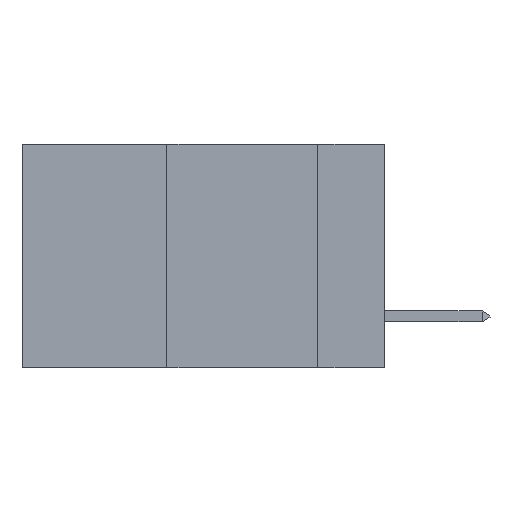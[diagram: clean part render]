
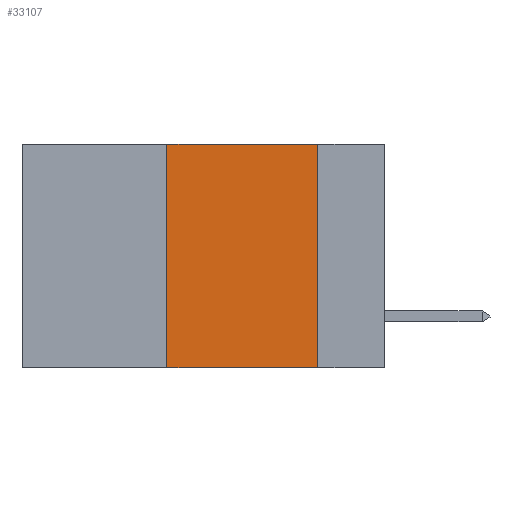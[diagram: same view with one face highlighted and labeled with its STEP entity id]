
A CAD part, left-side view. The second image highlights one B-rep face of the part: STEP entity #33107.
In plain terms, the highlighted planar face has unit normal (-1, 0, 0).
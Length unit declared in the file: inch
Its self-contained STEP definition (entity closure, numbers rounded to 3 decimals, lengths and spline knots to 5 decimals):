
#845 = CARTESIAN_POINT ( 'NONE',  ( 0., 0.6, -0.37 ) ) ;
#1303 = DIRECTION ( 'NONE',  ( 1., 0., 0. ) ) ;
#1881 = PLANE ( 'NONE',  #28845 ) ;
#2186 = CARTESIAN_POINT ( 'NONE',  ( 0., 0.11, -0.37 ) ) ;
#3560 = CARTESIAN_POINT ( 'NONE',  ( 0., 0.36, 0. ) ) ;
#4544 = DIRECTION ( 'NONE',  ( 0., -1., 0. ) ) ;
#4889 = DIRECTION ( 'NONE',  ( 0., 0., -1. ) ) ;
#6541 = EDGE_CURVE ( 'NONE', #30773, #9007, #35278, .T. ) ;
#7238 = DIRECTION ( 'NONE',  ( 0., -1., 0. ) ) ;
#7935 = CARTESIAN_POINT ( 'NONE',  ( 0., 0.36, 0. ) ) ;
#8057 = CARTESIAN_POINT ( 'NONE',  ( 0., 0.36, -0.37 ) ) ;
#8483 = EDGE_CURVE ( 'NONE', #10462, #10898, #13368, .T. ) ;
#9007 = VERTEX_POINT ( 'NONE', #2186 ) ;
#10462 = VERTEX_POINT ( 'NONE', #8057 ) ;
#10898 = VERTEX_POINT ( 'NONE', #3560 ) ;
#13368 = LINE ( 'NONE', #7935, #29173 ) ;
#14554 = VECTOR ( 'NONE', #4544, 39.37008 ) ;
#15826 = ORIENTED_EDGE ( 'NONE', *, *, #30664, .F. ) ;
#17549 = CARTESIAN_POINT ( 'NONE',  ( 0., 0.6, 0. ) ) ;
#18660 = EDGE_LOOP ( 'NONE', ( #22678, #15826, #23710, #25867 ) ) ;
#19678 = VECTOR ( 'NONE', #7238, 39.37008 ) ;
#20193 = LINE ( 'NONE', #40863, #14554 ) ;
#22678 = ORIENTED_EDGE ( 'NONE', *, *, #6541, .F. ) ;
#23710 = ORIENTED_EDGE ( 'NONE', *, *, #8483, .F. ) ;
#24102 = DIRECTION ( 'NONE',  ( 0., 0., -1. ) ) ;
#25867 = ORIENTED_EDGE ( 'NONE', *, *, #41255, .T. ) ;
#26531 = VECTOR ( 'NONE', #4889, 39.37008 ) ;
#28355 = LINE ( 'NONE', #845, #19678 ) ;
#28845 = AXIS2_PLACEMENT_3D ( 'NONE', #17549, #1303, #24102 ) ;
#29173 = VECTOR ( 'NONE', #30806, 39.37008 ) ;
#30548 = FACE_OUTER_BOUND ( 'NONE', #18660, .T. ) ;
#30664 = EDGE_CURVE ( 'NONE', #10898, #30773, #20193, .T. ) ;
#30773 = VERTEX_POINT ( 'NONE', #40989 ) ;
#30806 = DIRECTION ( 'NONE',  ( 0., 0., 1. ) ) ;
#33107 = ADVANCED_FACE ( 'NONE', ( #30548 ), #1881, .F. ) ;
#34883 = CARTESIAN_POINT ( 'NONE',  ( 0., 0.11, 0. ) ) ;
#35278 = LINE ( 'NONE', #34883, #26531 ) ;
#40863 = CARTESIAN_POINT ( 'NONE',  ( 0., 0.6, 0. ) ) ;
#40989 = CARTESIAN_POINT ( 'NONE',  ( 0., 0.11, 0. ) ) ;
#41255 = EDGE_CURVE ( 'NONE', #10462, #9007, #28355, .T. ) ;
